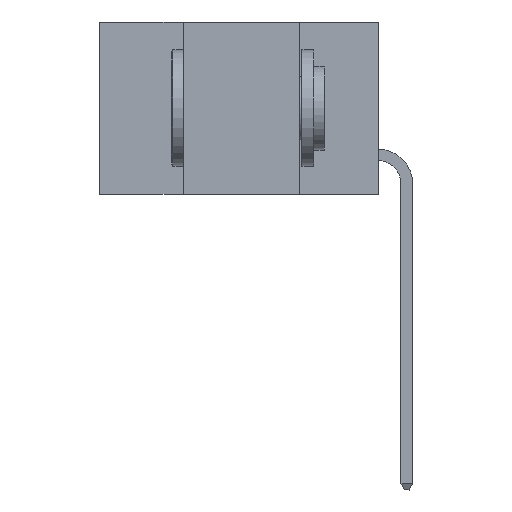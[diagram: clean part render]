
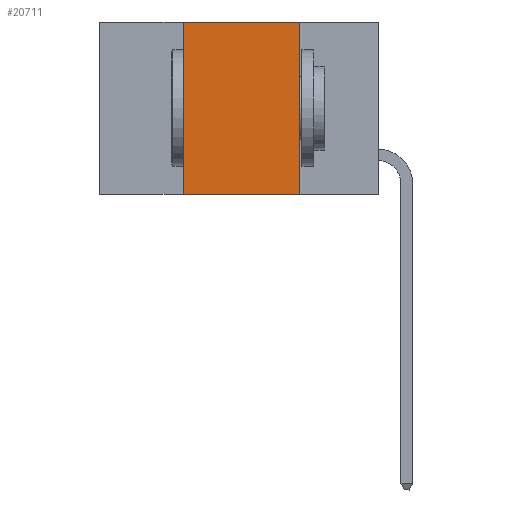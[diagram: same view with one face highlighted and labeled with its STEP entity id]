
A CAD part, left-side view. The second image highlights one B-rep face of the part: STEP entity #20711.
In plain terms, the highlighted planar face has unit normal (-1, 0, 0).
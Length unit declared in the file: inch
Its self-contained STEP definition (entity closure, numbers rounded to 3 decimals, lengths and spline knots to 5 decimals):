
#314 = ORIENTED_EDGE ( 'NONE', *, *, #6128, .F. ) ;
#495 = VERTEX_POINT ( 'NONE', #5324 ) ;
#1532 = ORIENTED_EDGE ( 'NONE', *, *, #4814, .F. ) ;
#2059 = LINE ( 'NONE', #10558, #2671 ) ;
#2186 = EDGE_CURVE ( 'NONE', #21004, #14879, #12979, .T. ) ;
#2624 = PLANE ( 'NONE',  #16826 ) ;
#2671 = VECTOR ( 'NONE', #10653, 39.37008 ) ;
#3605 = VERTEX_POINT ( 'NONE', #20738 ) ;
#3640 = FACE_OUTER_BOUND ( 'NONE', #9487, .T. ) ;
#4609 = DIRECTION ( 'NONE',  ( 1., 0., 0. ) ) ;
#4814 = EDGE_CURVE ( 'NONE', #21004, #3605, #11082, .T. ) ;
#5324 = CARTESIAN_POINT ( 'NONE',  ( 0., 0.17, 0. ) ) ;
#6128 = EDGE_CURVE ( 'NONE', #495, #14879, #2059, .T. ) ;
#6733 = ORIENTED_EDGE ( 'NONE', *, *, #2186, .T. ) ;
#7254 = VECTOR ( 'NONE', #19692, 39.37008 ) ;
#8094 = VECTOR ( 'NONE', #16532, 39.37008 ) ;
#9487 = EDGE_LOOP ( 'NONE', ( #314, #10537, #1532, #6733 ) ) ;
#10537 = ORIENTED_EDGE ( 'NONE', *, *, #21365, .F. ) ;
#10558 = CARTESIAN_POINT ( 'NONE',  ( 0., 0.17, 0. ) ) ;
#10617 = CARTESIAN_POINT ( 'NONE',  ( 0., 0.6, 0. ) ) ;
#10653 = DIRECTION ( 'NONE',  ( 0., 0., -1. ) ) ;
#11082 = LINE ( 'NONE', #16129, #20774 ) ;
#12979 = LINE ( 'NONE', #16257, #8094 ) ;
#14715 = CARTESIAN_POINT ( 'NONE',  ( 0., 0.42, -0.37 ) ) ;
#14879 = VERTEX_POINT ( 'NONE', #19211 ) ;
#16129 = CARTESIAN_POINT ( 'NONE',  ( 0., 0.42, 0. ) ) ;
#16257 = CARTESIAN_POINT ( 'NONE',  ( 0., 0.6, -0.37 ) ) ;
#16532 = DIRECTION ( 'NONE',  ( 0., -1., 0. ) ) ;
#16826 = AXIS2_PLACEMENT_3D ( 'NONE', #21147, #4609, #17612 ) ;
#17612 = DIRECTION ( 'NONE',  ( 0., 0., -1. ) ) ;
#18769 = DIRECTION ( 'NONE',  ( 0., 0., 1. ) ) ;
#19211 = CARTESIAN_POINT ( 'NONE',  ( 0., 0.17, -0.37 ) ) ;
#19692 = DIRECTION ( 'NONE',  ( 0., -1., 0. ) ) ;
#20711 = ADVANCED_FACE ( 'NONE', ( #3640 ), #2624, .F. ) ;
#20738 = CARTESIAN_POINT ( 'NONE',  ( 0., 0.42, 0. ) ) ;
#20774 = VECTOR ( 'NONE', #18769, 39.37008 ) ;
#21004 = VERTEX_POINT ( 'NONE', #14715 ) ;
#21147 = CARTESIAN_POINT ( 'NONE',  ( 0., 0.6, 0. ) ) ;
#21365 = EDGE_CURVE ( 'NONE', #3605, #495, #21837, .T. ) ;
#21837 = LINE ( 'NONE', #10617, #7254 ) ;
